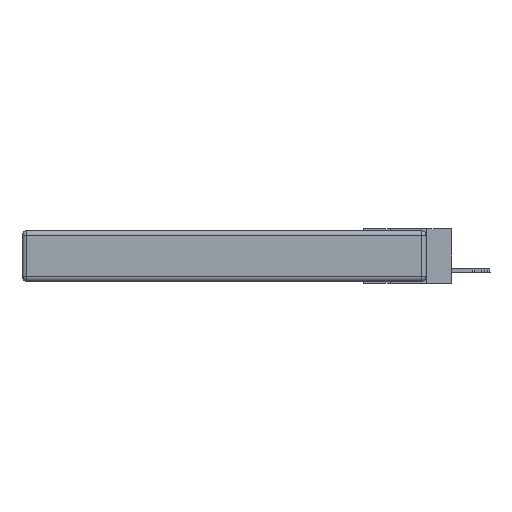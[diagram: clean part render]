
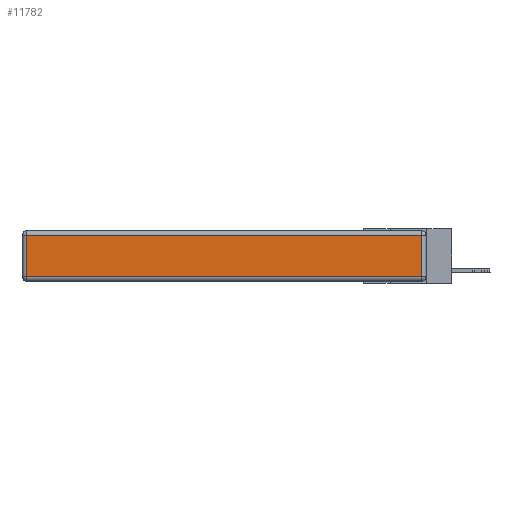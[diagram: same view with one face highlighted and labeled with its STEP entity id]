
A CAD part, left-side view. The second image highlights one B-rep face of the part: STEP entity #11782.
In plain terms, the highlighted planar face has unit normal (-1, 0, 0).
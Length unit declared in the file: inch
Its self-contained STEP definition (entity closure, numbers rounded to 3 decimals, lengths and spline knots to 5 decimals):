
#1576 = DIRECTION ( 'NONE',  ( 0., 0., -1. ) ) ;
#1865 = LINE ( 'NONE', #11914, #18066 ) ;
#2032 = EDGE_CURVE ( 'NONE', #8142, #3539, #3727, .T. ) ;
#2152 = VECTOR ( 'NONE', #2201, 39.37008 ) ;
#2201 = DIRECTION ( 'NONE',  ( 0., -1., 0. ) ) ;
#3347 = DIRECTION ( 'NONE',  ( 0., 1., 0. ) ) ;
#3539 = VERTEX_POINT ( 'NONE', #6699 ) ;
#3589 = LINE ( 'NONE', #16493, #7590 ) ;
#3727 = LINE ( 'NONE', #15985, #26707 ) ;
#6699 = CARTESIAN_POINT ( 'NONE',  ( 0., 2.72, -0.03 ) ) ;
#7590 = VECTOR ( 'NONE', #8763, 39.37008 ) ;
#8142 = VERTEX_POINT ( 'NONE', #11579 ) ;
#8763 = DIRECTION ( 'NONE',  ( 0., 0., 1. ) ) ;
#9088 = ORIENTED_EDGE ( 'NONE', *, *, #20570, .T. ) ;
#10965 = CARTESIAN_POINT ( 'NONE',  ( 0., 0., -0.343 ) ) ;
#11579 = CARTESIAN_POINT ( 'NONE',  ( 0., 0.03, -0.03 ) ) ;
#11782 = ADVANCED_FACE ( 'NONE', ( #16750 ), #13376, .T. ) ;
#11914 = CARTESIAN_POINT ( 'NONE',  ( 0., 2.72, -0.343 ) ) ;
#13376 = PLANE ( 'NONE',  #15224 ) ;
#14585 = ORIENTED_EDGE ( 'NONE', *, *, #32530, .T. ) ;
#14821 = LINE ( 'NONE', #30096, #2152 ) ;
#15224 = AXIS2_PLACEMENT_3D ( 'NONE', #10965, #28764, #31085 ) ;
#15985 = CARTESIAN_POINT ( 'NONE',  ( 0., 2.75, -0.03 ) ) ;
#16493 = CARTESIAN_POINT ( 'NONE',  ( 0., 0.03, -0.343 ) ) ;
#16750 = FACE_OUTER_BOUND ( 'NONE', #26635, .T. ) ;
#17666 = VERTEX_POINT ( 'NONE', #24800 ) ;
#17875 = VERTEX_POINT ( 'NONE', #18860 ) ;
#18066 = VECTOR ( 'NONE', #1576, 39.37008 ) ;
#18860 = CARTESIAN_POINT ( 'NONE',  ( 0., 2.72, -0.313 ) ) ;
#20570 = EDGE_CURVE ( 'NONE', #17666, #8142, #3589, .T. ) ;
#20947 = ORIENTED_EDGE ( 'NONE', *, *, #23267, .T. ) ;
#23267 = EDGE_CURVE ( 'NONE', #3539, #17875, #1865, .T. ) ;
#24800 = CARTESIAN_POINT ( 'NONE',  ( 0., 0.03, -0.313 ) ) ;
#26635 = EDGE_LOOP ( 'NONE', ( #14585, #9088, #27621, #20947 ) ) ;
#26707 = VECTOR ( 'NONE', #3347, 39.37008 ) ;
#27621 = ORIENTED_EDGE ( 'NONE', *, *, #2032, .T. ) ;
#28764 = DIRECTION ( 'NONE',  ( -1., 0., 0. ) ) ;
#30096 = CARTESIAN_POINT ( 'NONE',  ( 0., 0., -0.313 ) ) ;
#31085 = DIRECTION ( 'NONE',  ( 0., 0., 1. ) ) ;
#32530 = EDGE_CURVE ( 'NONE', #17875, #17666, #14821, .T. ) ;
